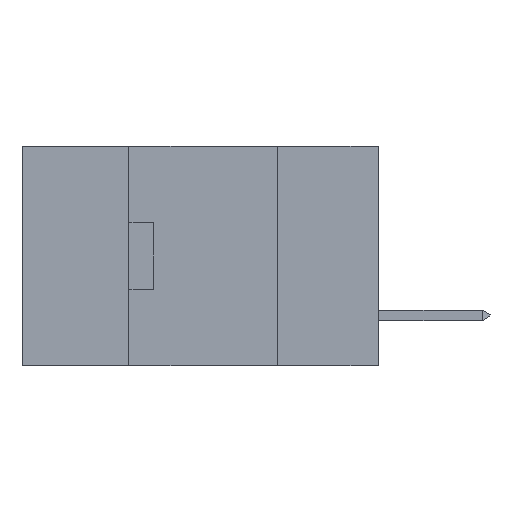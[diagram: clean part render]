
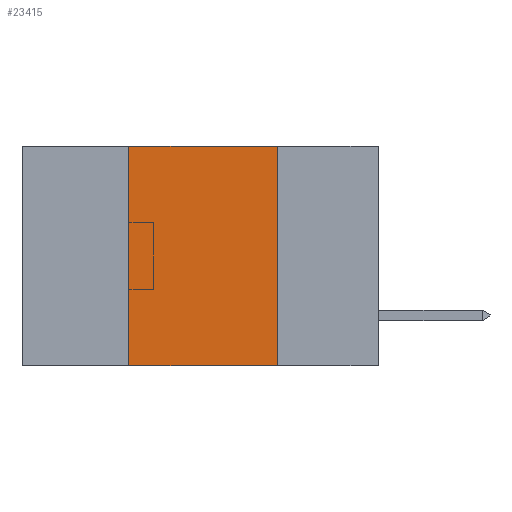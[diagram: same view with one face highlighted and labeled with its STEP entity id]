
A CAD part, left-side view. The second image highlights one B-rep face of the part: STEP entity #23415.
In plain terms, the highlighted planar face has unit normal (-1, 0, 0).
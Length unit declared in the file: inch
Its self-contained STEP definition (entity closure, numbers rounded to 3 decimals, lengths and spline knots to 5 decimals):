
#603 = CARTESIAN_POINT ( 'NONE',  ( 0., 0.17, -0.37 ) ) ;
#3325 = VERTEX_POINT ( 'NONE', #16321 ) ;
#3927 = VERTEX_POINT ( 'NONE', #5080 ) ;
#4382 = ORIENTED_EDGE ( 'NONE', *, *, #10527, .F. ) ;
#5080 = CARTESIAN_POINT ( 'NONE',  ( 0., 0.17, 0. ) ) ;
#7466 = DIRECTION ( 'NONE',  ( 1., 0., 0. ) ) ;
#7836 = VECTOR ( 'NONE', #17273, 39.37008 ) ;
#8186 = CARTESIAN_POINT ( 'NONE',  ( 0., 0.17, -0.37 ) ) ;
#8759 = EDGE_CURVE ( 'NONE', #11052, #26602, #20800, .T. ) ;
#9166 = VECTOR ( 'NONE', #20578, 39.37008 ) ;
#9260 = EDGE_LOOP ( 'NONE', ( #13200, #24006, #4382, #25997 ) ) ;
#9341 = LINE ( 'NONE', #17556, #7836 ) ;
#9494 = CARTESIAN_POINT ( 'NONE',  ( 0., 0.6, 0. ) ) ;
#10212 = LINE ( 'NONE', #8186, #9166 ) ;
#10390 = CARTESIAN_POINT ( 'NONE',  ( 0., 0.6, 0. ) ) ;
#10527 = EDGE_CURVE ( 'NONE', #11052, #3325, #9341, .T. ) ;
#11052 = VERTEX_POINT ( 'NONE', #15752 ) ;
#12329 = DIRECTION ( 'NONE',  ( 0., -1., 0. ) ) ;
#13066 = EDGE_CURVE ( 'NONE', #3927, #26602, #10212, .T. ) ;
#13200 = ORIENTED_EDGE ( 'NONE', *, *, #13066, .F. ) ;
#13228 = VECTOR ( 'NONE', #24951, 39.37008 ) ;
#15672 = FACE_OUTER_BOUND ( 'NONE', #9260, .T. ) ;
#15752 = CARTESIAN_POINT ( 'NONE',  ( 0., 0.42, -0.37 ) ) ;
#16321 = CARTESIAN_POINT ( 'NONE',  ( 0., 0.42, 0. ) ) ;
#17273 = DIRECTION ( 'NONE',  ( 0., 0., 1. ) ) ;
#17556 = CARTESIAN_POINT ( 'NONE',  ( 0., 0.42, -0.37 ) ) ;
#17705 = PLANE ( 'NONE',  #20161 ) ;
#20161 = AXIS2_PLACEMENT_3D ( 'NONE', #9494, #7466, #25812 ) ;
#20578 = DIRECTION ( 'NONE',  ( 0., 0., -1. ) ) ;
#20800 = LINE ( 'NONE', #22561, #21832 ) ;
#21832 = VECTOR ( 'NONE', #12329, 39.37008 ) ;
#22561 = CARTESIAN_POINT ( 'NONE',  ( 0., 0.6, -0.37 ) ) ;
#23415 = ADVANCED_FACE ( 'NONE', ( #15672 ), #17705, .F. ) ;
#24006 = ORIENTED_EDGE ( 'NONE', *, *, #24275, .F. ) ;
#24275 = EDGE_CURVE ( 'NONE', #3325, #3927, #24818, .T. ) ;
#24818 = LINE ( 'NONE', #10390, #13228 ) ;
#24951 = DIRECTION ( 'NONE',  ( 0., -1., 0. ) ) ;
#25812 = DIRECTION ( 'NONE',  ( 0., 0., -1. ) ) ;
#25997 = ORIENTED_EDGE ( 'NONE', *, *, #8759, .T. ) ;
#26602 = VERTEX_POINT ( 'NONE', #603 ) ;
